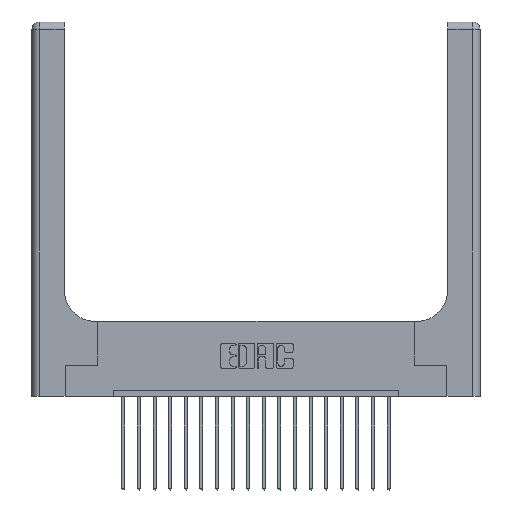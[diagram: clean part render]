
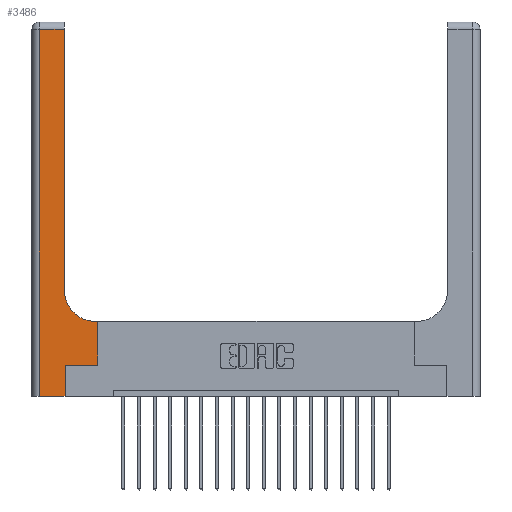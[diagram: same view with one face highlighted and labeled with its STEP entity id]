
A CAD part, top view. The second image highlights one B-rep face of the part: STEP entity #3486.
In plain terms, the highlighted planar face has unit normal (0, 0, 1).
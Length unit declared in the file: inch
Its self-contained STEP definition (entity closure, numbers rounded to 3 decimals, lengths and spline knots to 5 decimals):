
#178 = CARTESIAN_POINT ( 'NONE',  ( 0.265, 0.25, 0.37 ) ) ;
#308 = CIRCLE ( 'NONE', #8846, 0.25 ) ;
#789 = CARTESIAN_POINT ( 'NONE',  ( 0.06, 2.94, 0.37 ) ) ;
#1117 = ORIENTED_EDGE ( 'NONE', *, *, #8165, .T. ) ;
#1218 = VECTOR ( 'NONE', #1923, 39.37008 ) ;
#1442 = ORIENTED_EDGE ( 'NONE', *, *, #18048, .T. ) ;
#1923 = DIRECTION ( 'NONE',  ( 0., 1., 0. ) ) ;
#2056 = EDGE_CURVE ( 'NONE', #2521, #19244, #14955, .T. ) ;
#2077 = CARTESIAN_POINT ( 'NONE',  ( 0.26, 0.6, 0.37 ) ) ;
#2285 = ORIENTED_EDGE ( 'NONE', *, *, #7462, .T. ) ;
#2295 = DIRECTION ( 'NONE',  ( 0., 0., -1. ) ) ;
#2521 = VERTEX_POINT ( 'NONE', #19107 ) ;
#2680 = LINE ( 'NONE', #13243, #11649 ) ;
#2829 = LINE ( 'NONE', #16134, #12518 ) ;
#2841 = ORIENTED_EDGE ( 'NONE', *, *, #12781, .T. ) ;
#3126 = LINE ( 'NONE', #17265, #3824 ) ;
#3484 = VECTOR ( 'NONE', #10048, 39.37008 ) ;
#3486 = ADVANCED_FACE ( 'NONE', ( #16846 ), #17374, .F. ) ;
#3586 = DIRECTION ( 'NONE',  ( -1., 0., 0. ) ) ;
#3620 = LINE ( 'NONE', #2077, #4770 ) ;
#3824 = VECTOR ( 'NONE', #15551, 39.37008 ) ;
#4253 = VERTEX_POINT ( 'NONE', #5798 ) ;
#4354 = ORIENTED_EDGE ( 'NONE', *, *, #8532, .T. ) ;
#4770 = VECTOR ( 'NONE', #3586, 39.37008 ) ;
#4957 = AXIS2_PLACEMENT_3D ( 'NONE', #14289, #2295, #5174 ) ;
#5094 = CARTESIAN_POINT ( 'NONE',  ( 0.528, 0.25, 0.37 ) ) ;
#5130 = VERTEX_POINT ( 'NONE', #8606 ) ;
#5159 = CARTESIAN_POINT ( 'NONE',  ( 0.26, 0.85, 0.37 ) ) ;
#5174 = DIRECTION ( 'NONE',  ( -1., 0., 0. ) ) ;
#5563 = CARTESIAN_POINT ( 'NONE',  ( 0.26, 3., 0.37 ) ) ;
#5798 = CARTESIAN_POINT ( 'NONE',  ( 0.26, 2.94, 0.37 ) ) ;
#5857 = DIRECTION ( 'NONE',  ( 1., 0., 0. ) ) ;
#6572 = CARTESIAN_POINT ( 'NONE',  ( 0.06, 0., 0.37 ) ) ;
#7462 = EDGE_CURVE ( 'NONE', #19489, #12992, #2680, .T. ) ;
#7957 = CARTESIAN_POINT ( 'NONE',  ( 0.51, 0.6, 0.37 ) ) ;
#8165 = EDGE_CURVE ( 'NONE', #4253, #19489, #3126, .T. ) ;
#8532 = EDGE_CURVE ( 'NONE', #16171, #8695, #308, .T. ) ;
#8606 = CARTESIAN_POINT ( 'NONE',  ( 0.265, 0., 0.37 ) ) ;
#8685 = LINE ( 'NONE', #5563, #3484 ) ;
#8695 = VERTEX_POINT ( 'NONE', #5159 ) ;
#8846 = AXIS2_PLACEMENT_3D ( 'NONE', #13814, #16887, #15284 ) ;
#10048 = DIRECTION ( 'NONE',  ( 0., 1., 0. ) ) ;
#10499 = CARTESIAN_POINT ( 'NONE',  ( 0.265, 0., 0.37 ) ) ;
#11415 = EDGE_CURVE ( 'NONE', #12992, #5130, #2829, .T. ) ;
#11649 = VECTOR ( 'NONE', #17645, 39.37008 ) ;
#11901 = DIRECTION ( 'NONE',  ( 0., 1., 0. ) ) ;
#12187 = CARTESIAN_POINT ( 'NONE',  ( 0.265, 0.25, 0.37 ) ) ;
#12518 = VECTOR ( 'NONE', #13185, 39.37008 ) ;
#12781 = EDGE_CURVE ( 'NONE', #16595, #2521, #14605, .T. ) ;
#12931 = LINE ( 'NONE', #10499, #14600 ) ;
#12992 = VERTEX_POINT ( 'NONE', #6572 ) ;
#13185 = DIRECTION ( 'NONE',  ( 1., 0., 0. ) ) ;
#13243 = CARTESIAN_POINT ( 'NONE',  ( 0.06, 3., 0.37 ) ) ;
#13814 = CARTESIAN_POINT ( 'NONE',  ( 0.51, 0.85, 0.37 ) ) ;
#13823 = CARTESIAN_POINT ( 'NONE',  ( 0.528, 0.6, 0.37 ) ) ;
#14289 = CARTESIAN_POINT ( 'NONE',  ( 0., 3., 0.37 ) ) ;
#14316 = EDGE_LOOP ( 'NONE', ( #14334, #1117, #2285, #18890, #1442, #2841, #18155, #15298, #4354 ) ) ;
#14334 = ORIENTED_EDGE ( 'NONE', *, *, #17148, .T. ) ;
#14600 = VECTOR ( 'NONE', #11901, 39.37008 ) ;
#14605 = LINE ( 'NONE', #12187, #16041 ) ;
#14955 = LINE ( 'NONE', #5094, #1218 ) ;
#15284 = DIRECTION ( 'NONE',  ( 1., 0., 0. ) ) ;
#15298 = ORIENTED_EDGE ( 'NONE', *, *, #15606, .T. ) ;
#15551 = DIRECTION ( 'NONE',  ( -1., 0., 0. ) ) ;
#15606 = EDGE_CURVE ( 'NONE', #19244, #16171, #3620, .T. ) ;
#16041 = VECTOR ( 'NONE', #5857, 39.37008 ) ;
#16134 = CARTESIAN_POINT ( 'NONE',  ( 0., 0., 0.37 ) ) ;
#16171 = VERTEX_POINT ( 'NONE', #7957 ) ;
#16595 = VERTEX_POINT ( 'NONE', #178 ) ;
#16846 = FACE_OUTER_BOUND ( 'NONE', #14316, .T. ) ;
#16887 = DIRECTION ( 'NONE',  ( 0., 0., -1. ) ) ;
#17148 = EDGE_CURVE ( 'NONE', #8695, #4253, #8685, .T. ) ;
#17265 = CARTESIAN_POINT ( 'NONE',  ( 0., 2.94, 0.37 ) ) ;
#17374 = PLANE ( 'NONE',  #4957 ) ;
#17645 = DIRECTION ( 'NONE',  ( 0., -1., 0. ) ) ;
#18048 = EDGE_CURVE ( 'NONE', #5130, #16595, #12931, .T. ) ;
#18155 = ORIENTED_EDGE ( 'NONE', *, *, #2056, .T. ) ;
#18890 = ORIENTED_EDGE ( 'NONE', *, *, #11415, .T. ) ;
#19107 = CARTESIAN_POINT ( 'NONE',  ( 0.528, 0.25, 0.37 ) ) ;
#19244 = VERTEX_POINT ( 'NONE', #13823 ) ;
#19489 = VERTEX_POINT ( 'NONE', #789 ) ;
